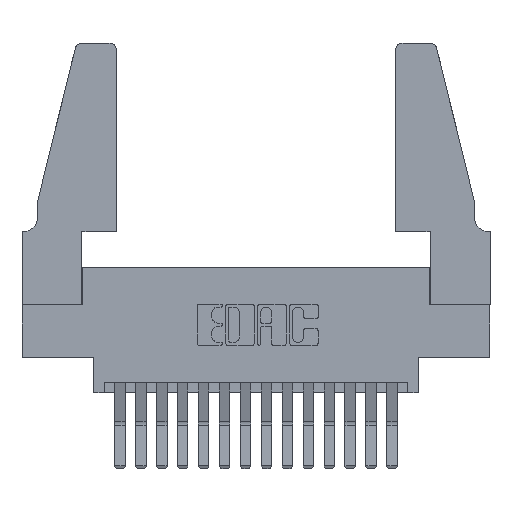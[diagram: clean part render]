
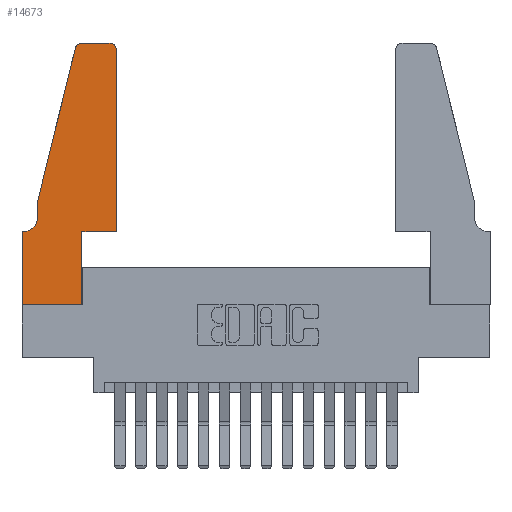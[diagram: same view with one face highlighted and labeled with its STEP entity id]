
A CAD part, top view. The second image highlights one B-rep face of the part: STEP entity #14673.
In plain terms, the highlighted planar face has unit normal (0, 0, 1).
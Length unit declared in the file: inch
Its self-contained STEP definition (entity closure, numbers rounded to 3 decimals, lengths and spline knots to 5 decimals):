
#47 = LINE ( 'NONE', #12559, #5869 ) ;
#88 = CARTESIAN_POINT ( 'NONE',  ( 0., 0., 0.37 ) ) ;
#107 = CARTESIAN_POINT ( 'NONE',  ( 0.0755, 0.42, 0.37 ) ) ;
#313 = CARTESIAN_POINT ( 'NONE',  ( 0.4505, 0.35, 0.37 ) ) ;
#484 = VERTEX_POINT ( 'NONE', #107 ) ;
#570 = VERTEX_POINT ( 'NONE', #16198 ) ;
#1016 = DIRECTION ( 'NONE',  ( 0., 0., -1. ) ) ;
#1159 = ORIENTED_EDGE ( 'NONE', *, *, #8601, .T. ) ;
#1368 = AXIS2_PLACEMENT_3D ( 'NONE', #6236, #1016, #7688 ) ;
#1429 = LINE ( 'NONE', #2408, #8711 ) ;
#1443 = DIRECTION ( 'NONE',  ( 0., -1., 0. ) ) ;
#1505 = CARTESIAN_POINT ( 'NONE',  ( 0.2865, 0.35, 0.37 ) ) ;
#1688 = VERTEX_POINT ( 'NONE', #15975 ) ;
#1872 = CARTESIAN_POINT ( 'NONE',  ( 0., 0., 0.37 ) ) ;
#2080 = CARTESIAN_POINT ( 'NONE',  ( 0., 0.35, 0.37 ) ) ;
#2181 = EDGE_CURVE ( 'NONE', #570, #3849, #6897, .T. ) ;
#2231 = EDGE_CURVE ( 'NONE', #484, #4127, #12043, .T. ) ;
#2331 = CARTESIAN_POINT ( 'NONE',  ( 0.25487, 1.22718, 0.37 ) ) ;
#2368 = EDGE_CURVE ( 'NONE', #6658, #13705, #12244, .T. ) ;
#2408 = CARTESIAN_POINT ( 'NONE',  ( 0.0755, 0.5, 0.37 ) ) ;
#2452 = DIRECTION ( 'NONE',  ( 1., 0., 0. ) ) ;
#2606 = PLANE ( 'NONE',  #12070 ) ;
#2687 = VERTEX_POINT ( 'NONE', #12498 ) ;
#2939 = EDGE_CURVE ( 'NONE', #4127, #10918, #12425, .T. ) ;
#3640 = EDGE_CURVE ( 'NONE', #13705, #13637, #1429, .T. ) ;
#3786 = VECTOR ( 'NONE', #10940, 39.37008 ) ;
#3805 = CARTESIAN_POINT ( 'NONE',  ( 0.0755, 0.35, 0.37 ) ) ;
#3849 = VERTEX_POINT ( 'NONE', #13502 ) ;
#3931 = ORIENTED_EDGE ( 'NONE', *, *, #2368, .T. ) ;
#4127 = VERTEX_POINT ( 'NONE', #6197 ) ;
#4548 = ORIENTED_EDGE ( 'NONE', *, *, #2181, .T. ) ;
#5098 = DIRECTION ( 'NONE',  ( 0., 1., 0. ) ) ;
#5259 = DIRECTION ( 'NONE',  ( 0., 0., 1. ) ) ;
#5281 = DIRECTION ( 'NONE',  ( 0., 0., 1. ) ) ;
#5577 = VERTEX_POINT ( 'NONE', #1872 ) ;
#5815 = CARTESIAN_POINT ( 'NONE',  ( 0.2605, 1.25, 0.37 ) ) ;
#5869 = VECTOR ( 'NONE', #7332, 39.37008 ) ;
#5898 = VERTEX_POINT ( 'NONE', #14877 ) ;
#5961 = LINE ( 'NONE', #11980, #11105 ) ;
#6124 = DIRECTION ( 'NONE',  ( 1., 0., 0. ) ) ;
#6197 = CARTESIAN_POINT ( 'NONE',  ( 0.0055, 0.35, 0.37 ) ) ;
#6208 = CARTESIAN_POINT ( 'NONE',  ( 0.4505, 0.35, 0.37 ) ) ;
#6235 = ORIENTED_EDGE ( 'NONE', *, *, #16073, .T. ) ;
#6236 = CARTESIAN_POINT ( 'NONE',  ( 0.0055, 0.42, 0.37 ) ) ;
#6658 = VERTEX_POINT ( 'NONE', #15910 ) ;
#6792 = DIRECTION ( 'NONE',  ( 1., 0., 0. ) ) ;
#6897 = LINE ( 'NONE', #313, #11639 ) ;
#7332 = DIRECTION ( 'NONE',  ( 1., 0., 0. ) ) ;
#7688 = DIRECTION ( 'NONE',  ( -1., 0., 0. ) ) ;
#7834 = ORIENTED_EDGE ( 'NONE', *, *, #2231, .T. ) ;
#7910 = CIRCLE ( 'NONE', #13872, 0.03 ) ;
#7954 = CARTESIAN_POINT ( 'NONE',  ( 0., 0.35, 0.37 ) ) ;
#8061 = EDGE_LOOP ( 'NONE', ( #9112, #3931, #14414, #14196, #7834, #16879, #1159, #8261, #6235, #4548, #9865, #10111 ) ) ;
#8261 = ORIENTED_EDGE ( 'NONE', *, *, #14213, .T. ) ;
#8601 = EDGE_CURVE ( 'NONE', #10918, #5577, #9685, .T. ) ;
#8711 = VECTOR ( 'NONE', #11784, 39.37008 ) ;
#8868 = CARTESIAN_POINT ( 'NONE',  ( 0.0755, 0.5, 0.37 ) ) ;
#9112 = ORIENTED_EDGE ( 'NONE', *, *, #14011, .T. ) ;
#9115 = VECTOR ( 'NONE', #12216, 39.37008 ) ;
#9240 = DIRECTION ( 'NONE',  ( 0., 0., 1. ) ) ;
#9373 = DIRECTION ( 'NONE',  ( 0., -1., 0. ) ) ;
#9461 = VECTOR ( 'NONE', #5098, 39.37008 ) ;
#9618 = VECTOR ( 'NONE', #9373, 39.37008 ) ;
#9685 = LINE ( 'NONE', #88, #9618 ) ;
#9865 = ORIENTED_EDGE ( 'NONE', *, *, #16996, .T. ) ;
#10111 = ORIENTED_EDGE ( 'NONE', *, *, #15245, .T. ) ;
#10496 = CARTESIAN_POINT ( 'NONE',  ( 0.4205, 1.22, 0.37 ) ) ;
#10918 = VERTEX_POINT ( 'NONE', #2080 ) ;
#10940 = DIRECTION ( 'NONE',  ( -1., 0., 0. ) ) ;
#11105 = VECTOR ( 'NONE', #1443, 39.37008 ) ;
#11112 = EDGE_CURVE ( 'NONE', #13637, #484, #5961, .T. ) ;
#11556 = LINE ( 'NONE', #1505, #9115 ) ;
#11639 = VECTOR ( 'NONE', #6124, 39.37008 ) ;
#11771 = DIRECTION ( 'NONE',  ( -1., 0., 0. ) ) ;
#11784 = DIRECTION ( 'NONE',  ( -0.239, -0.971, 0. ) ) ;
#11980 = CARTESIAN_POINT ( 'NONE',  ( 0.0755, 0.5, 0.37 ) ) ;
#12043 = CIRCLE ( 'NONE', #1368, 0.07 ) ;
#12070 = AXIS2_PLACEMENT_3D ( 'NONE', #7954, #5281, #6792 ) ;
#12216 = DIRECTION ( 'NONE',  ( 0., 1., 0. ) ) ;
#12244 = CIRCLE ( 'NONE', #13788, 0.03 ) ;
#12425 = LINE ( 'NONE', #3805, #15550 ) ;
#12498 = CARTESIAN_POINT ( 'NONE',  ( 0.2865, 0., 0.37 ) ) ;
#12559 = CARTESIAN_POINT ( 'NONE',  ( 0., 0., 0.37 ) ) ;
#13502 = CARTESIAN_POINT ( 'NONE',  ( 0.4505, 0.35, 0.37 ) ) ;
#13637 = VERTEX_POINT ( 'NONE', #8868 ) ;
#13705 = VERTEX_POINT ( 'NONE', #2331 ) ;
#13788 = AXIS2_PLACEMENT_3D ( 'NONE', #15825, #9240, #17084 ) ;
#13872 = AXIS2_PLACEMENT_3D ( 'NONE', #10496, #5259, #2452 ) ;
#14011 = EDGE_CURVE ( 'NONE', #1688, #6658, #15790, .T. ) ;
#14196 = ORIENTED_EDGE ( 'NONE', *, *, #11112, .T. ) ;
#14213 = EDGE_CURVE ( 'NONE', #5577, #2687, #47, .T. ) ;
#14414 = ORIENTED_EDGE ( 'NONE', *, *, #3640, .T. ) ;
#14673 = ADVANCED_FACE ( 'NONE', ( #15384 ), #2606, .T. ) ;
#14877 = CARTESIAN_POINT ( 'NONE',  ( 0.4505, 1.22, 0.37 ) ) ;
#15245 = EDGE_CURVE ( 'NONE', #5898, #1688, #7910, .T. ) ;
#15384 = FACE_OUTER_BOUND ( 'NONE', #8061, .T. ) ;
#15550 = VECTOR ( 'NONE', #11771, 39.37008 ) ;
#15790 = LINE ( 'NONE', #5815, #3786 ) ;
#15825 = CARTESIAN_POINT ( 'NONE',  ( 0.284, 1.22, 0.37 ) ) ;
#15910 = CARTESIAN_POINT ( 'NONE',  ( 0.284, 1.25, 0.37 ) ) ;
#15975 = CARTESIAN_POINT ( 'NONE',  ( 0.4205, 1.25, 0.37 ) ) ;
#16073 = EDGE_CURVE ( 'NONE', #2687, #570, #11556, .T. ) ;
#16198 = CARTESIAN_POINT ( 'NONE',  ( 0.2865, 0.35, 0.37 ) ) ;
#16291 = LINE ( 'NONE', #6208, #9461 ) ;
#16879 = ORIENTED_EDGE ( 'NONE', *, *, #2939, .T. ) ;
#16996 = EDGE_CURVE ( 'NONE', #3849, #5898, #16291, .T. ) ;
#17084 = DIRECTION ( 'NONE',  ( 1., 0., 0. ) ) ;
